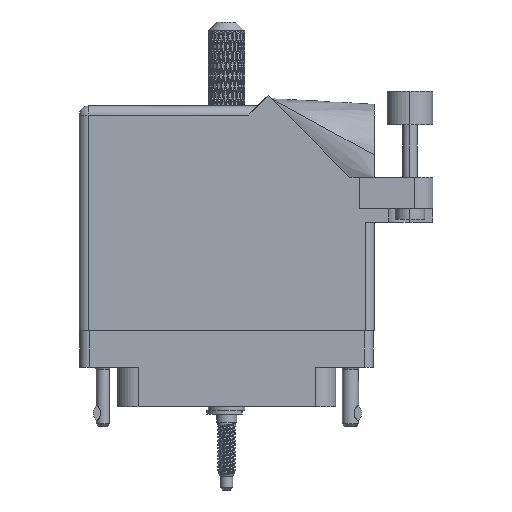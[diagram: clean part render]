
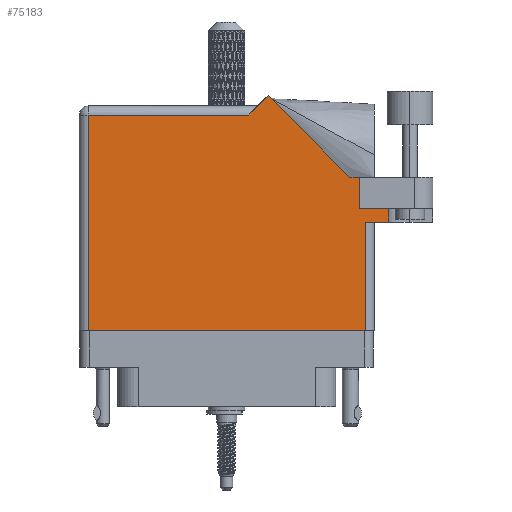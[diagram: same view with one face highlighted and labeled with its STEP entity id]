
A CAD part, front view. The second image highlights one B-rep face of the part: STEP entity #75183.
In plain terms, the highlighted face is planar.
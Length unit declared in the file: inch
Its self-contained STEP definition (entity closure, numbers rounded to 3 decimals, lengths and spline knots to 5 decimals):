
#1868 = ORIENTED_EDGE ( 'NONE', *, *, #38105, .T. ) ;
#2685 = CARTESIAN_POINT ( 'NONE',  ( -1.005, 1.43, 0.455 ) ) ;
#3083 = DIRECTION ( 'NONE',  ( 0., 0., -1. ) ) ;
#4546 = VERTEX_POINT ( 'NONE', #68103 ) ;
#4561 = ORIENTED_EDGE ( 'NONE', *, *, #106386, .T. ) ;
#5061 = CARTESIAN_POINT ( 'NONE',  ( -0.943, -0.1, 0.455 ) ) ;
#7906 = EDGE_CURVE ( 'NONE', #46142, #99613, #89376, .T. ) ;
#8514 = EDGE_LOOP ( 'NONE', ( #111432, #107018, #100116, #14712, #48178, #4561, #73473, #34742, #57437, #38483, #1868 ) ) ;
#9840 = CARTESIAN_POINT ( 'NONE',  ( 1.1065, 0.637, 0.455 ) ) ;
#10610 = CARTESIAN_POINT ( 'NONE',  ( 0.83942, 0.944, 0.455 ) ) ;
#11342 = VECTOR ( 'NONE', #72548, 39.37008 ) ;
#12357 = LINE ( 'NONE', #109349, #40296 ) ;
#12394 = VERTEX_POINT ( 'NONE', #87133 ) ;
#12410 = PLANE ( 'NONE',  #107666 ) ;
#14712 = ORIENTED_EDGE ( 'NONE', *, *, #65301, .F. ) ;
#15514 = CARTESIAN_POINT ( 'NONE',  ( 1.005, 0.637, 0.455 ) ) ;
#18308 = LINE ( 'NONE', #10610, #11342 ) ;
#18857 = CARTESIAN_POINT ( 'NONE',  ( 1.1065, 1.06177, 0.455 ) ) ;
#23035 = DIRECTION ( 'NONE',  ( 1., 0., 0. ) ) ;
#23112 = DIRECTION ( 'NONE',  ( -1., 0., 0. ) ) ;
#24183 = CARTESIAN_POINT ( 'NONE',  ( 0.905, 0.731, 0.455 ) ) ;
#26836 = FACE_OUTER_BOUND ( 'NONE', #8514, .T. ) ;
#27515 = EDGE_CURVE ( 'NONE', #102976, #4546, #12357, .T. ) ;
#30700 = CARTESIAN_POINT ( 'NONE',  ( 0.943, -0.1, 0.455 ) ) ;
#30842 = VERTEX_POINT ( 'NONE', #79130 ) ;
#31208 = CARTESIAN_POINT ( 'NONE',  ( -1.005, -0.1, 0.455 ) ) ;
#32945 = CARTESIAN_POINT ( 'NONE',  ( 0.212, 1.43, 0.455 ) ) ;
#33056 = CARTESIAN_POINT ( 'NONE',  ( 0.905, 0.944, 0.455 ) ) ;
#34061 = DIRECTION ( 'NONE',  ( -1., 0., 0. ) ) ;
#34742 = ORIENTED_EDGE ( 'NONE', *, *, #56738, .T. ) ;
#35906 = LINE ( 'NONE', #18857, #88861 ) ;
#36742 = VECTOR ( 'NONE', #95474, 39.37008 ) ;
#37755 = CARTESIAN_POINT ( 'NONE',  ( 0.83942, 0.944, 0.455 ) ) ;
#38105 = EDGE_CURVE ( 'NONE', #68341, #50925, #57638, .T. ) ;
#38483 = ORIENTED_EDGE ( 'NONE', *, *, #104734, .T. ) ;
#40296 = VECTOR ( 'NONE', #46374, 39.37008 ) ;
#44572 = VECTOR ( 'NONE', #23035, 39.37008 ) ;
#45835 = CARTESIAN_POINT ( 'NONE',  ( 0.15, 1.368, 0.455 ) ) ;
#46142 = VERTEX_POINT ( 'NONE', #33056 ) ;
#46374 = DIRECTION ( 'NONE',  ( 0., 1., 0. ) ) ;
#48178 = ORIENTED_EDGE ( 'NONE', *, *, #94261, .F. ) ;
#50925 = VERTEX_POINT ( 'NONE', #5061 ) ;
#52947 = LINE ( 'NONE', #24183, #44572 ) ;
#56216 = LINE ( 'NONE', #31208, #77146 ) ;
#56346 = DIRECTION ( 'NONE',  ( -0.707, -0.707, 0. ) ) ;
#56738 = EDGE_CURVE ( 'NONE', #99613, #79893, #18308, .T. ) ;
#57337 = VECTOR ( 'NONE', #23112, 39.37008 ) ;
#57404 = DIRECTION ( 'NONE',  ( 0., 1., 0. ) ) ;
#57437 = ORIENTED_EDGE ( 'NONE', *, *, #107570, .T. ) ;
#57638 = LINE ( 'NONE', #68198, #36742 ) ;
#65301 = EDGE_CURVE ( 'NONE', #30842, #88041, #35906, .T. ) ;
#67608 = CARTESIAN_POINT ( 'NONE',  ( -1.005, 1.368, 0.455 ) ) ;
#68103 = CARTESIAN_POINT ( 'NONE',  ( 0.943, 0.637, 0.455 ) ) ;
#68198 = CARTESIAN_POINT ( 'NONE',  ( -0.943, -0.1, 0.455 ) ) ;
#68341 = VERTEX_POINT ( 'NONE', #94915 ) ;
#72548 = DIRECTION ( 'NONE',  ( -0.707, 0.707, 0. ) ) ;
#73473 = ORIENTED_EDGE ( 'NONE', *, *, #7906, .T. ) ;
#73735 = LINE ( 'NONE', #93630, #109888 ) ;
#74718 = EDGE_CURVE ( 'NONE', #50925, #102976, #56216, .T. ) ;
#75183 = ADVANCED_FACE ( 'NONE', ( #26836 ), #12410, .F. ) ;
#76837 = EDGE_CURVE ( 'NONE', #4546, #88041, #106037, .T. ) ;
#76985 = VERTEX_POINT ( 'NONE', #45835 ) ;
#77056 = DIRECTION ( 'NONE',  ( 1., 0., 0. ) ) ;
#77146 = VECTOR ( 'NONE', #94741, 39.37008 ) ;
#77783 = LINE ( 'NONE', #32945, #83383 ) ;
#79130 = CARTESIAN_POINT ( 'NONE',  ( 1.1065, 0.731, 0.455 ) ) ;
#79893 = VERTEX_POINT ( 'NONE', #89048 ) ;
#80817 = DIRECTION ( 'NONE',  ( 0., -1., 0. ) ) ;
#82430 = VECTOR ( 'NONE', #77056, 39.37008 ) ;
#82972 = DIRECTION ( 'NONE',  ( -1., 0., 0. ) ) ;
#83383 = VECTOR ( 'NONE', #56346, 39.37008 ) ;
#85038 = CARTESIAN_POINT ( 'NONE',  ( 1.405, 0.944, 0.455 ) ) ;
#87133 = CARTESIAN_POINT ( 'NONE',  ( 0.905, 0.731, 0.455 ) ) ;
#88041 = VERTEX_POINT ( 'NONE', #9840 ) ;
#88861 = VECTOR ( 'NONE', #80817, 39.37008 ) ;
#89048 = CARTESIAN_POINT ( 'NONE',  ( 0.28271, 1.50071, 0.455 ) ) ;
#89376 = LINE ( 'NONE', #85038, #57337 ) ;
#93630 = CARTESIAN_POINT ( 'NONE',  ( 0.905, 0.731, 0.455 ) ) ;
#94261 = EDGE_CURVE ( 'NONE', #12394, #30842, #52947, .T. ) ;
#94730 = LINE ( 'NONE', #67608, #97504 ) ;
#94741 = DIRECTION ( 'NONE',  ( 1., 0., 0. ) ) ;
#94915 = CARTESIAN_POINT ( 'NONE',  ( -0.943, 1.368, 0.455 ) ) ;
#95474 = DIRECTION ( 'NONE',  ( 0., -1., 0. ) ) ;
#97504 = VECTOR ( 'NONE', #34061, 39.37008 ) ;
#99613 = VERTEX_POINT ( 'NONE', #37755 ) ;
#100116 = ORIENTED_EDGE ( 'NONE', *, *, #76837, .T. ) ;
#102976 = VERTEX_POINT ( 'NONE', #30700 ) ;
#104734 = EDGE_CURVE ( 'NONE', #76985, #68341, #94730, .T. ) ;
#106037 = LINE ( 'NONE', #15514, #82430 ) ;
#106386 = EDGE_CURVE ( 'NONE', #12394, #46142, #73735, .T. ) ;
#107018 = ORIENTED_EDGE ( 'NONE', *, *, #27515, .T. ) ;
#107570 = EDGE_CURVE ( 'NONE', #79893, #76985, #77783, .T. ) ;
#107666 = AXIS2_PLACEMENT_3D ( 'NONE', #2685, #3083, #82972 ) ;
#109349 = CARTESIAN_POINT ( 'NONE',  ( 0.943, 0.637, 0.455 ) ) ;
#109888 = VECTOR ( 'NONE', #57404, 39.37008 ) ;
#111432 = ORIENTED_EDGE ( 'NONE', *, *, #74718, .T. ) ;
